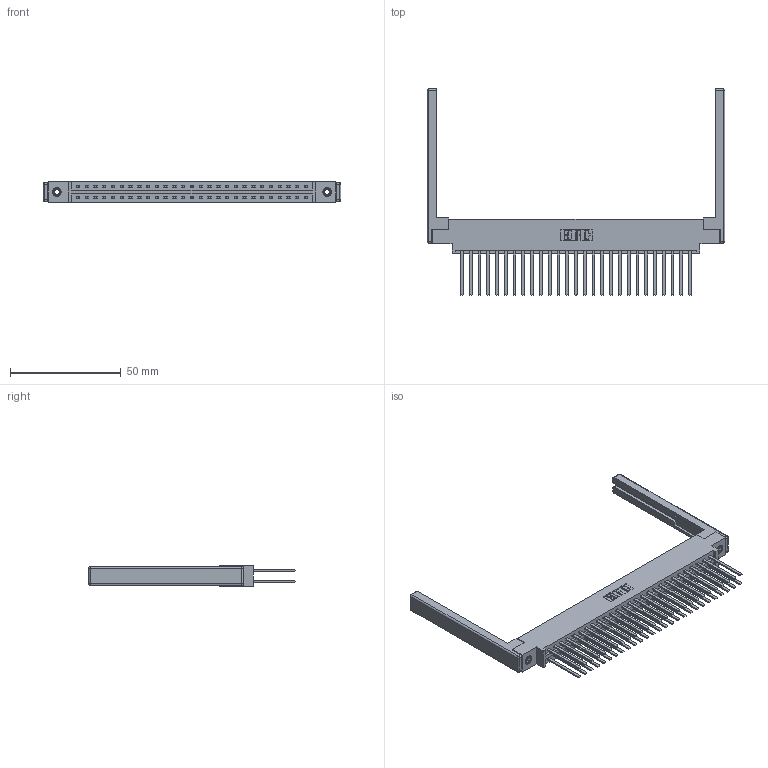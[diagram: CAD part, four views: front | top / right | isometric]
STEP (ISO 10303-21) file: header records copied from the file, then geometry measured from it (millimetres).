
FILE_DESCRIPTION (( 'STEP AP203' ), '1' );
FILE_NAME ('387-054-544-868.STEP', '2019-10-19T05:22:54', ( '' ), ( '' ), 'SwSTEP 2.0', 'SolidWorks 2016', '' );
FILE_SCHEMA (( 'CONFIG_CONTROL_DESIGN' ));
Length unit declared in the file: inch
Products named in the file (5): 345-292-001_345-293-144; 307-220-068; 387-054-544-868; 345-250-001_345-250-001-102; 337 Part_0.170 Offset - 0.156 Dia-TI
Assembly tree (59 placements, depth 2):
  387-054-544-868
    337 Part_0.170 Offset - 0.156 Dia-TI
    345-292-001_345-293-144  x54
    345-250-001_345-250-001-102  x2
    307-220-068  x2
Bounding box: 134.42 x 93.35 x 9.4 mm (x, y, z)
Volume: 18990.5 mm3; surface area: 22981.1 mm2
Topology: 59 solids, 59 shells, 2864 faces, 8435 edges, 5530 vertices
Faces by surface type: plane 1998, cylinder 842, cone 12, sphere 8, torus 4
Entity records: 25582 total; most frequent: CARTESIAN_POINT 4287, ORIENTED_EDGE 4212, DIRECTION 3740, EDGE_CURVE 2106, LINE 1932, VECTOR 1932, VERTEX_POINT 1394, AXIS2_PLACEMENT_3D 904
